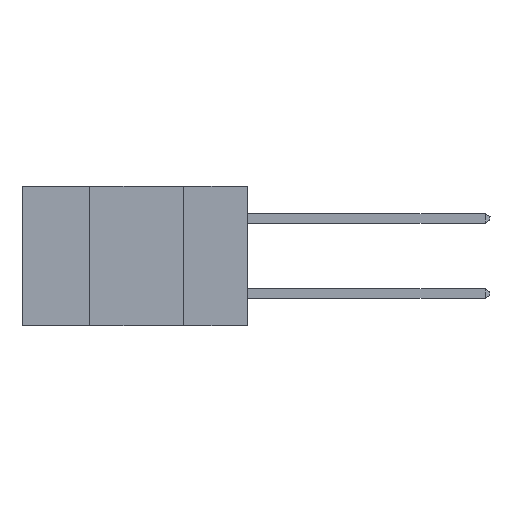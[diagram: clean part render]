
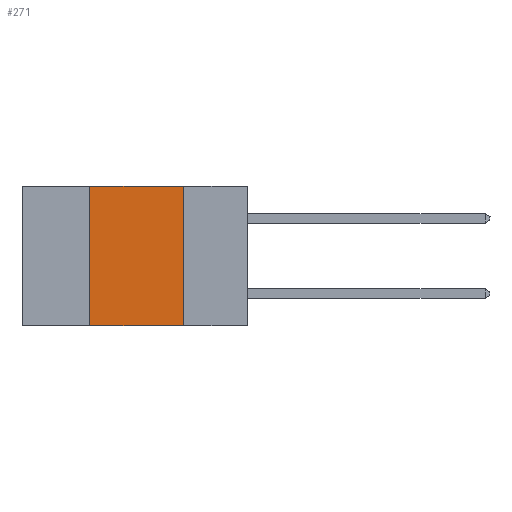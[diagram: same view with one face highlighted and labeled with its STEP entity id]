
A CAD part, left-side view. The second image highlights one B-rep face of the part: STEP entity #271.
In plain terms, the highlighted planar face has unit normal (-1, 0, 0).
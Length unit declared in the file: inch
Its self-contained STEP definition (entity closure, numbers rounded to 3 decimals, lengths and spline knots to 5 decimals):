
#8 = LINE ( 'NONE', #1598, #2214 ) ;
#201 = VECTOR ( 'NONE', #7125, 39.37008 ) ;
#219 = VERTEX_POINT ( 'NONE', #2052 ) ;
#271 = ADVANCED_FACE ( 'NONE', ( #5767 ), #3948, .F. ) ;
#669 = VERTEX_POINT ( 'NONE', #3136 ) ;
#942 = CARTESIAN_POINT ( 'NONE',  ( 0., 0.17, 0. ) ) ;
#1022 = CARTESIAN_POINT ( 'NONE',  ( 0., 0.17, -0.37 ) ) ;
#1557 = ORIENTED_EDGE ( 'NONE', *, *, #8579, .F. ) ;
#1598 = CARTESIAN_POINT ( 'NONE',  ( 0., 0.6, -0.37 ) ) ;
#1653 = AXIS2_PLACEMENT_3D ( 'NONE', #8411, #10896, #4937 ) ;
#2026 = EDGE_CURVE ( 'NONE', #669, #10857, #8, .T. ) ;
#2052 = CARTESIAN_POINT ( 'NONE',  ( 0., 0.17, 0. ) ) ;
#2214 = VECTOR ( 'NONE', #4093, 39.37008 ) ;
#2459 = EDGE_CURVE ( 'NONE', #6380, #219, #9715, .T. ) ;
#3136 = CARTESIAN_POINT ( 'NONE',  ( 0., 0.42, -0.37 ) ) ;
#3948 = PLANE ( 'NONE',  #1653 ) ;
#4005 = CARTESIAN_POINT ( 'NONE',  ( 0., 0.42, 0. ) ) ;
#4093 = DIRECTION ( 'NONE',  ( 0., -1., 0. ) ) ;
#4533 = LINE ( 'NONE', #942, #201 ) ;
#4830 = EDGE_CURVE ( 'NONE', #669, #6380, #10891, .T. ) ;
#4937 = DIRECTION ( 'NONE',  ( 0., 0., -1. ) ) ;
#5767 = FACE_OUTER_BOUND ( 'NONE', #5971, .T. ) ;
#5971 = EDGE_LOOP ( 'NONE', ( #1557, #8286, #6788, #9606 ) ) ;
#5979 = VECTOR ( 'NONE', #9874, 39.37008 ) ;
#6380 = VERTEX_POINT ( 'NONE', #6771 ) ;
#6771 = CARTESIAN_POINT ( 'NONE',  ( 0., 0.42, 0. ) ) ;
#6788 = ORIENTED_EDGE ( 'NONE', *, *, #4830, .F. ) ;
#7125 = DIRECTION ( 'NONE',  ( 0., 0., -1. ) ) ;
#7177 = CARTESIAN_POINT ( 'NONE',  ( 0., 0.6, 0. ) ) ;
#7652 = DIRECTION ( 'NONE',  ( 0., 0., 1. ) ) ;
#8151 = VECTOR ( 'NONE', #7652, 39.37008 ) ;
#8286 = ORIENTED_EDGE ( 'NONE', *, *, #2459, .F. ) ;
#8411 = CARTESIAN_POINT ( 'NONE',  ( 0., 0.6, 0. ) ) ;
#8579 = EDGE_CURVE ( 'NONE', #219, #10857, #4533, .T. ) ;
#9606 = ORIENTED_EDGE ( 'NONE', *, *, #2026, .T. ) ;
#9715 = LINE ( 'NONE', #7177, #5979 ) ;
#9874 = DIRECTION ( 'NONE',  ( 0., -1., 0. ) ) ;
#10857 = VERTEX_POINT ( 'NONE', #1022 ) ;
#10891 = LINE ( 'NONE', #4005, #8151 ) ;
#10896 = DIRECTION ( 'NONE',  ( 1., 0., 0. ) ) ;
